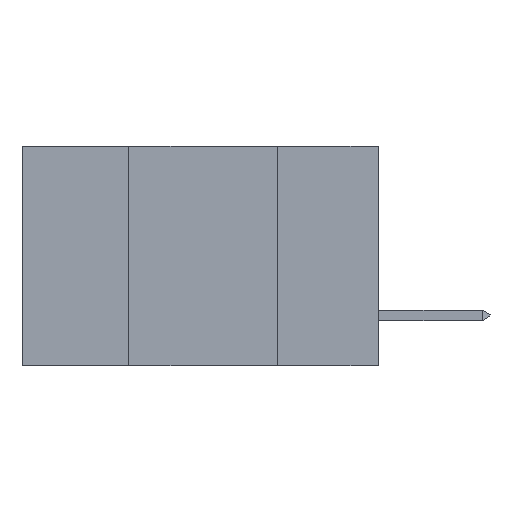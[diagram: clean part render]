
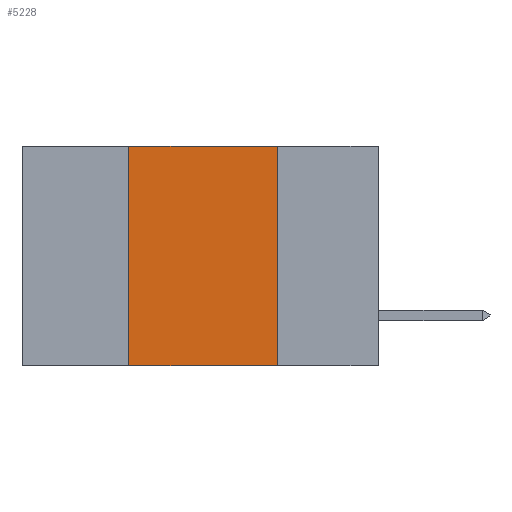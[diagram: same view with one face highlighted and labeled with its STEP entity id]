
A CAD part, left-side view. The second image highlights one B-rep face of the part: STEP entity #5228.
In plain terms, the highlighted planar face has unit normal (-1, 0, 0).
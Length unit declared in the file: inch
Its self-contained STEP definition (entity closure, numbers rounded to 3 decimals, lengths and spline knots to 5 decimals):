
#1274 = CARTESIAN_POINT ( 'NONE',  ( 0., 0.6, 0. ) ) ;
#2183 = VERTEX_POINT ( 'NONE', #7302 ) ;
#2415 = DIRECTION ( 'NONE',  ( 1., 0., 0. ) ) ;
#3439 = VECTOR ( 'NONE', #9945, 39.37008 ) ;
#3532 = CARTESIAN_POINT ( 'NONE',  ( 0., 0.42, -0.37 ) ) ;
#3628 = CARTESIAN_POINT ( 'NONE',  ( 0., 0.42, -0.37 ) ) ;
#3935 = CARTESIAN_POINT ( 'NONE',  ( 0., 0.17, -0.37 ) ) ;
#4924 = LINE ( 'NONE', #1274, #6426 ) ;
#5101 = CARTESIAN_POINT ( 'NONE',  ( 0., 0.17, 0. ) ) ;
#5138 = CARTESIAN_POINT ( 'NONE',  ( 0., 0.6, 0. ) ) ;
#5228 = ADVANCED_FACE ( 'NONE', ( #10548 ), #9649, .F. ) ;
#5364 = LINE ( 'NONE', #3532, #3439 ) ;
#5484 = ORIENTED_EDGE ( 'NONE', *, *, #9906, .F. ) ;
#5847 = DIRECTION ( 'NONE',  ( 0., 0., -1. ) ) ;
#5927 = EDGE_LOOP ( 'NONE', ( #11334, #5484, #7907, #8442 ) ) ;
#6063 = DIRECTION ( 'NONE',  ( 0., -1., 0. ) ) ;
#6426 = VECTOR ( 'NONE', #9336, 39.37008 ) ;
#6909 = EDGE_CURVE ( 'NONE', #8765, #8063, #5364, .T. ) ;
#7199 = EDGE_CURVE ( 'NONE', #8765, #2183, #9693, .T. ) ;
#7220 = VECTOR ( 'NONE', #6063, 39.37008 ) ;
#7302 = CARTESIAN_POINT ( 'NONE',  ( 0., 0.17, -0.37 ) ) ;
#7544 = DIRECTION ( 'NONE',  ( 0., 0., -1. ) ) ;
#7724 = CARTESIAN_POINT ( 'NONE',  ( 0., 0.6, -0.37 ) ) ;
#7907 = ORIENTED_EDGE ( 'NONE', *, *, #6909, .F. ) ;
#8063 = VERTEX_POINT ( 'NONE', #8391 ) ;
#8378 = LINE ( 'NONE', #3935, #8500 ) ;
#8391 = CARTESIAN_POINT ( 'NONE',  ( 0., 0.42, 0. ) ) ;
#8442 = ORIENTED_EDGE ( 'NONE', *, *, #7199, .T. ) ;
#8500 = VECTOR ( 'NONE', #7544, 39.37008 ) ;
#8765 = VERTEX_POINT ( 'NONE', #3628 ) ;
#9336 = DIRECTION ( 'NONE',  ( 0., -1., 0. ) ) ;
#9649 = PLANE ( 'NONE',  #10264 ) ;
#9693 = LINE ( 'NONE', #7724, #7220 ) ;
#9886 = EDGE_CURVE ( 'NONE', #9965, #2183, #8378, .T. ) ;
#9906 = EDGE_CURVE ( 'NONE', #8063, #9965, #4924, .T. ) ;
#9945 = DIRECTION ( 'NONE',  ( 0., 0., 1. ) ) ;
#9965 = VERTEX_POINT ( 'NONE', #5101 ) ;
#10264 = AXIS2_PLACEMENT_3D ( 'NONE', #5138, #2415, #5847 ) ;
#10548 = FACE_OUTER_BOUND ( 'NONE', #5927, .T. ) ;
#11334 = ORIENTED_EDGE ( 'NONE', *, *, #9886, .F. ) ;
